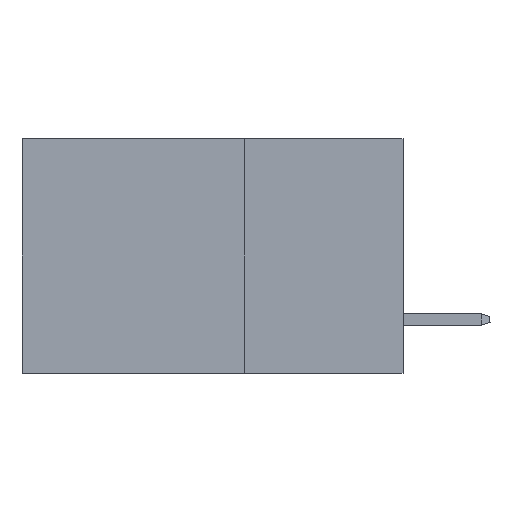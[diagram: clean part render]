
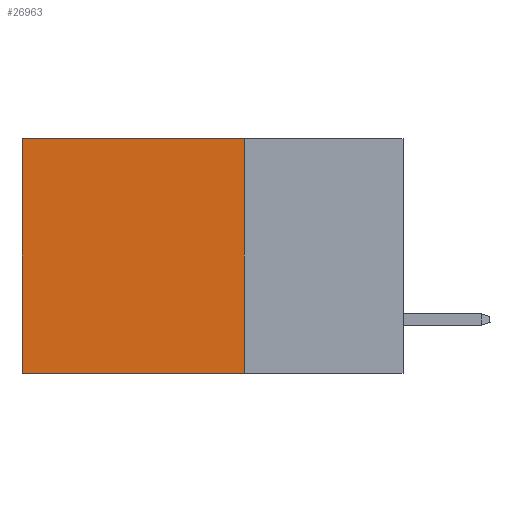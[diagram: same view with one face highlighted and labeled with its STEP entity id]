
A CAD part, left-side view. The second image highlights one B-rep face of the part: STEP entity #26963.
In plain terms, the highlighted planar face has unit normal (-1, 0, 0).
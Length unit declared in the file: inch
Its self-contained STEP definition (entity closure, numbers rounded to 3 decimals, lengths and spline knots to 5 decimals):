
#1456 = VERTEX_POINT ( 'NONE', #35559 ) ;
#2795 = CARTESIAN_POINT ( 'NONE',  ( 0.2875, 0.6, 0. ) ) ;
#3727 = DIRECTION ( 'NONE',  ( 0., 0., -1. ) ) ;
#4070 = ORIENTED_EDGE ( 'NONE', *, *, #29701, .T. ) ;
#5530 = LINE ( 'NONE', #11081, #37135 ) ;
#8158 = ORIENTED_EDGE ( 'NONE', *, *, #27436, .T. ) ;
#9710 = DIRECTION ( 'NONE',  ( 0., 1., 0. ) ) ;
#10251 = VECTOR ( 'NONE', #9710, 39.37008 ) ;
#10500 = CARTESIAN_POINT ( 'NONE',  ( 0.2875, 0.25, 0. ) ) ;
#11081 = CARTESIAN_POINT ( 'NONE',  ( 0.2875, 0.25, -0.37 ) ) ;
#13813 = VECTOR ( 'NONE', #30655, 39.37008 ) ;
#14149 = DIRECTION ( 'NONE',  ( 0., 1., 0. ) ) ;
#18315 = DIRECTION ( 'NONE',  ( 1., 0., 0. ) ) ;
#18990 = DIRECTION ( 'NONE',  ( 0., 0., -1. ) ) ;
#21156 = VERTEX_POINT ( 'NONE', #28332 ) ;
#21175 = AXIS2_PLACEMENT_3D ( 'NONE', #29825, #18315, #3727 ) ;
#21250 = EDGE_CURVE ( 'NONE', #30404, #1456, #31211, .T. ) ;
#22133 = EDGE_CURVE ( 'NONE', #1456, #21156, #5530, .T. ) ;
#23784 = CARTESIAN_POINT ( 'NONE',  ( 0.2875, 0.25, 0. ) ) ;
#26963 = ADVANCED_FACE ( 'NONE', ( #27135 ), #32696, .F. ) ;
#27135 = FACE_OUTER_BOUND ( 'NONE', #28402, .T. ) ;
#27436 = EDGE_CURVE ( 'NONE', #31346, #21156, #35314, .T. ) ;
#28332 = CARTESIAN_POINT ( 'NONE',  ( 0.2875, 0.6, -0.37 ) ) ;
#28402 = EDGE_LOOP ( 'NONE', ( #8158, #36869, #32996, #4070 ) ) ;
#29701 = EDGE_CURVE ( 'NONE', #30404, #31346, #33295, .T. ) ;
#29825 = CARTESIAN_POINT ( 'NONE',  ( 0.2875, 0.25, 0. ) ) ;
#30059 = CARTESIAN_POINT ( 'NONE',  ( 0.2875, 0.25, 0. ) ) ;
#30404 = VERTEX_POINT ( 'NONE', #23784 ) ;
#30655 = DIRECTION ( 'NONE',  ( 0., 0., -1. ) ) ;
#31211 = LINE ( 'NONE', #10500, #13813 ) ;
#31346 = VERTEX_POINT ( 'NONE', #2795 ) ;
#32696 = PLANE ( 'NONE',  #21175 ) ;
#32996 = ORIENTED_EDGE ( 'NONE', *, *, #21250, .F. ) ;
#33295 = LINE ( 'NONE', #30059, #10251 ) ;
#35314 = LINE ( 'NONE', #36407, #37695 ) ;
#35559 = CARTESIAN_POINT ( 'NONE',  ( 0.2875, 0.25, -0.37 ) ) ;
#36407 = CARTESIAN_POINT ( 'NONE',  ( 0.2875, 0.6, 0. ) ) ;
#36869 = ORIENTED_EDGE ( 'NONE', *, *, #22133, .F. ) ;
#37135 = VECTOR ( 'NONE', #14149, 39.37008 ) ;
#37695 = VECTOR ( 'NONE', #18990, 39.37008 ) ;
